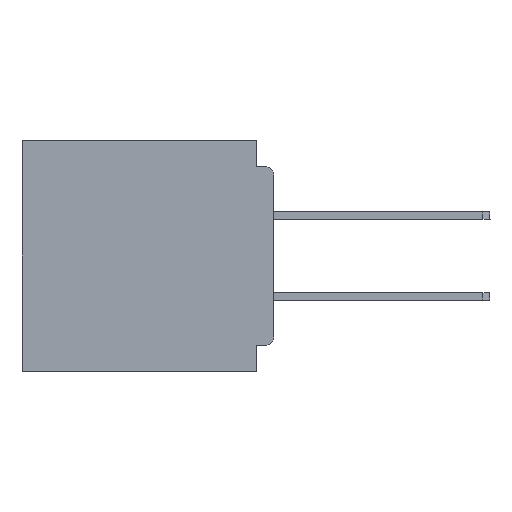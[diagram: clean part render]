
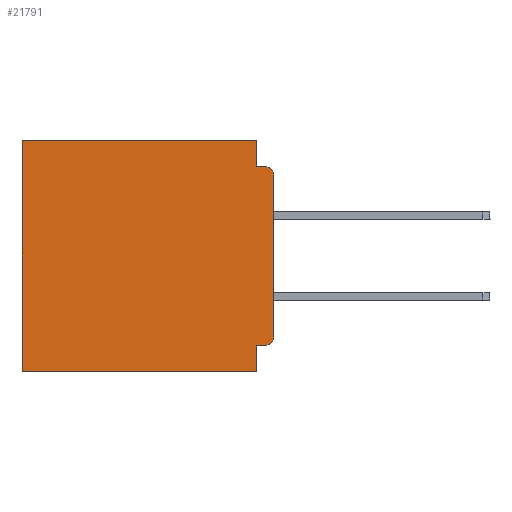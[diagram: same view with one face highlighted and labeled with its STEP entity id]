
A CAD part, left-side view. The second image highlights one B-rep face of the part: STEP entity #21791.
In plain terms, the highlighted planar face has unit normal (-1, 0, 0).
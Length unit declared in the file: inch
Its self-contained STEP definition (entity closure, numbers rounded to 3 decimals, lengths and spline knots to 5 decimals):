
#357 = DIRECTION ( 'NONE',  ( -1., 0., 0. ) ) ;
#1362 = ORIENTED_EDGE ( 'NONE', *, *, #56263, .F. ) ;
#2084 = CARTESIAN_POINT ( 'NONE',  ( 0.3, 0.437, 0. ) ) ;
#2672 = CARTESIAN_POINT ( 'NONE',  ( 0.3, 0.437, -0.4 ) ) ;
#2742 = CARTESIAN_POINT ( 'NONE',  ( 0.3, 0., -0.4 ) ) ;
#2951 = CARTESIAN_POINT ( 'NONE',  ( 0.3, 0.031, 0. ) ) ;
#2970 = LINE ( 'NONE', #48472, #38188 ) ;
#3350 = VECTOR ( 'NONE', #18122, 39.37008 ) ;
#3680 = AXIS2_PLACEMENT_3D ( 'NONE', #2742, #37746, #7832 ) ;
#4083 = CARTESIAN_POINT ( 'NONE',  ( 0.3, 0.015, -0.045 ) ) ;
#4924 = LINE ( 'NONE', #2951, #3350 ) ;
#6415 = VERTEX_POINT ( 'NONE', #2084 ) ;
#7832 = DIRECTION ( 'NONE',  ( 0., 0., -1. ) ) ;
#9800 = VERTEX_POINT ( 'NONE', #29818 ) ;
#10209 = VERTEX_POINT ( 'NONE', #63609 ) ;
#10280 = EDGE_CURVE ( 'NONE', #61820, #6415, #58585, .T. ) ;
#10639 = VERTEX_POINT ( 'NONE', #51898 ) ;
#11964 = CARTESIAN_POINT ( 'NONE',  ( 0.3, 0.015, -0.34 ) ) ;
#13027 = LINE ( 'NONE', #27454, #51252 ) ;
#13657 = DIRECTION ( 'NONE',  ( 0., 1., 0. ) ) ;
#14466 = CARTESIAN_POINT ( 'NONE',  ( 0.3, 0., 0. ) ) ;
#16843 = ORIENTED_EDGE ( 'NONE', *, *, #25697, .F. ) ;
#17027 = VECTOR ( 'NONE', #27279, 39.37008 ) ;
#17035 = DIRECTION ( 'NONE',  ( 0., 0., -1. ) ) ;
#17062 = EDGE_CURVE ( 'NONE', #9800, #40263, #13027, .T. ) ;
#17350 = VECTOR ( 'NONE', #54331, 39.37008 ) ;
#18122 = DIRECTION ( 'NONE',  ( 0., 0., -1. ) ) ;
#18594 = EDGE_CURVE ( 'NONE', #41833, #37143, #42605, .T. ) ;
#20736 = VECTOR ( 'NONE', #37676, 39.37008 ) ;
#21791 = ADVANCED_FACE ( 'NONE', ( #31264 ), #57511, .F. ) ;
#22305 = LINE ( 'NONE', #2672, #20736 ) ;
#22664 = AXIS2_PLACEMENT_3D ( 'NONE', #11964, #46823, #17035 ) ;
#22814 = ORIENTED_EDGE ( 'NONE', *, *, #53380, .F. ) ;
#23198 = LINE ( 'NONE', #37255, #17027 ) ;
#24370 = EDGE_CURVE ( 'NONE', #6415, #57088, #22305, .T. ) ;
#24920 = ORIENTED_EDGE ( 'NONE', *, *, #18594, .F. ) ;
#25697 = EDGE_CURVE ( 'NONE', #61820, #41833, #4924, .T. ) ;
#25714 = CARTESIAN_POINT ( 'NONE',  ( 0.3, 0.015, -0.355 ) ) ;
#27279 = DIRECTION ( 'NONE',  ( 0., 0., -1. ) ) ;
#27454 = CARTESIAN_POINT ( 'NONE',  ( 0.3, 0., -0.4 ) ) ;
#28983 = VERTEX_POINT ( 'NONE', #25714 ) ;
#29657 = ORIENTED_EDGE ( 'NONE', *, *, #48227, .F. ) ;
#29818 = CARTESIAN_POINT ( 'NONE',  ( 0.3, 0., -0.06 ) ) ;
#30015 = EDGE_CURVE ( 'NONE', #9800, #37143, #63869, .T. ) ;
#30409 = CARTESIAN_POINT ( 'NONE',  ( 0.3, 0.015, -0.06 ) ) ;
#31264 = FACE_OUTER_BOUND ( 'NONE', #54559, .T. ) ;
#32408 = ORIENTED_EDGE ( 'NONE', *, *, #30015, .T. ) ;
#32490 = CARTESIAN_POINT ( 'NONE',  ( 0.3, 0., -0.34 ) ) ;
#32508 = CARTESIAN_POINT ( 'NONE',  ( 0.3, 0.031, 0. ) ) ;
#35196 = LINE ( 'NONE', #43547, #46831 ) ;
#35366 = DIRECTION ( 'NONE',  ( 0., 0., -1. ) ) ;
#37143 = VERTEX_POINT ( 'NONE', #4083 ) ;
#37255 = CARTESIAN_POINT ( 'NONE',  ( 0.3, 0.031, -0.4 ) ) ;
#37676 = DIRECTION ( 'NONE',  ( 0., 0., -1. ) ) ;
#37746 = DIRECTION ( 'NONE',  ( 1., 0., 0. ) ) ;
#38188 = VECTOR ( 'NONE', #38687, 39.37008 ) ;
#38687 = DIRECTION ( 'NONE',  ( 0., 1., 0. ) ) ;
#40263 = VERTEX_POINT ( 'NONE', #32490 ) ;
#41152 = ORIENTED_EDGE ( 'NONE', *, *, #47397, .T. ) ;
#41833 = VERTEX_POINT ( 'NONE', #42860 ) ;
#42605 = LINE ( 'NONE', #47269, #54262 ) ;
#42860 = CARTESIAN_POINT ( 'NONE',  ( 0.3, 0.031, -0.045 ) ) ;
#43547 = CARTESIAN_POINT ( 'NONE',  ( 0.3, 0., -0.355 ) ) ;
#46343 = ORIENTED_EDGE ( 'NONE', *, *, #17062, .F. ) ;
#46823 = DIRECTION ( 'NONE',  ( -1., 0., 0. ) ) ;
#46831 = VECTOR ( 'NONE', #13657, 39.37008 ) ;
#47269 = CARTESIAN_POINT ( 'NONE',  ( 0.3, 0., -0.045 ) ) ;
#47397 = EDGE_CURVE ( 'NONE', #28983, #40263, #49964, .T. ) ;
#48227 = EDGE_CURVE ( 'NONE', #10209, #57088, #2970, .T. ) ;
#48472 = CARTESIAN_POINT ( 'NONE',  ( 0.3, 0., -0.4 ) ) ;
#49964 = CIRCLE ( 'NONE', #22664, 0.015 ) ;
#51252 = VECTOR ( 'NONE', #62169, 39.37008 ) ;
#51898 = CARTESIAN_POINT ( 'NONE',  ( 0.3, 0.031, -0.355 ) ) ;
#52291 = DIRECTION ( 'NONE',  ( 0., -1., 0. ) ) ;
#52540 = AXIS2_PLACEMENT_3D ( 'NONE', #30409, #357, #35366 ) ;
#52730 = ORIENTED_EDGE ( 'NONE', *, *, #10280, .T. ) ;
#53380 = EDGE_CURVE ( 'NONE', #28983, #10639, #35196, .T. ) ;
#54262 = VECTOR ( 'NONE', #52291, 39.37008 ) ;
#54331 = DIRECTION ( 'NONE',  ( 0., 1., 0. ) ) ;
#54559 = EDGE_LOOP ( 'NONE', ( #46343, #32408, #24920, #16843, #52730, #63145, #29657, #1362, #22814, #41152 ) ) ;
#56263 = EDGE_CURVE ( 'NONE', #10639, #10209, #23198, .T. ) ;
#57088 = VERTEX_POINT ( 'NONE', #63831 ) ;
#57511 = PLANE ( 'NONE',  #3680 ) ;
#58585 = LINE ( 'NONE', #14466, #17350 ) ;
#61820 = VERTEX_POINT ( 'NONE', #32508 ) ;
#62169 = DIRECTION ( 'NONE',  ( 0., 0., -1. ) ) ;
#63145 = ORIENTED_EDGE ( 'NONE', *, *, #24370, .T. ) ;
#63609 = CARTESIAN_POINT ( 'NONE',  ( 0.3, 0.031, -0.4 ) ) ;
#63831 = CARTESIAN_POINT ( 'NONE',  ( 0.3, 0.437, -0.4 ) ) ;
#63869 = CIRCLE ( 'NONE', #52540, 0.015 ) ;
